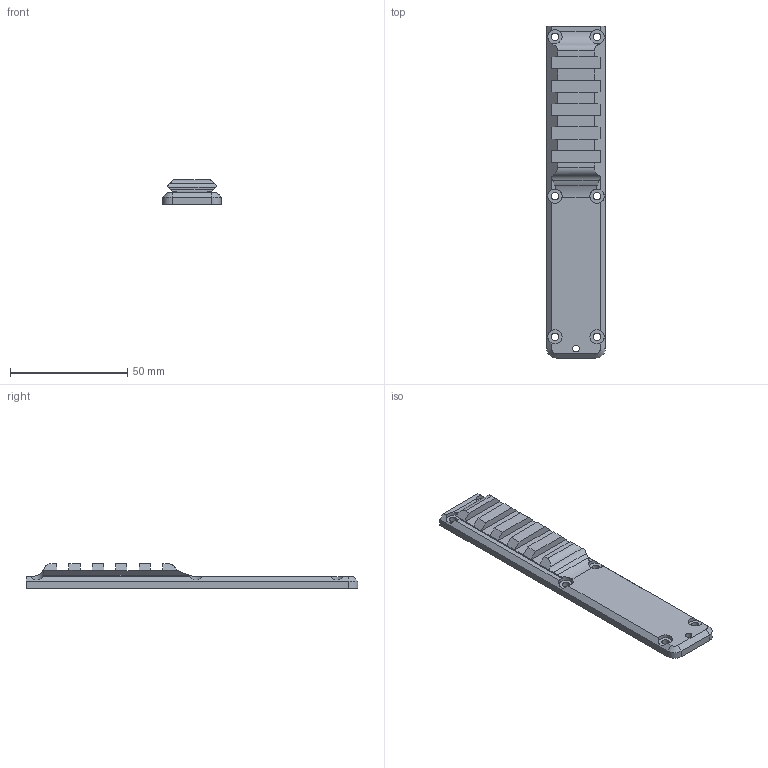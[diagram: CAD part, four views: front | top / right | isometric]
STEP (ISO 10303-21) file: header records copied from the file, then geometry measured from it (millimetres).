
FILE_DESCRIPTION(/* description */ (''),/* implementation_level */ '2;1');
FILE_NAME(/* name */ 'Receiver-Top-Cover_Picatinny.stp',/* time_stamp */ '2020-10-15T21:28:55-05:00',/* author */ (''),/* organization */ (''),/* preprocessor_version */ 'ST-DEVELOPER v15.2',/* originating_system */ 'Autodesk Translator Framework v2.0.0.5431',/* authorisation */ '');
FILE_SCHEMA (('AUTOMOTIVE_DESIGN { 1 0 10303 214 3 1 1 }'));
Length unit declared in the file: centimetre
Products named in the file (1): Receiver-Top-Cover_Picatinny
Bounding box: 25 x 141.66 x 10.47 mm (x, y, z)
Volume: 16500.9 mm3; surface area: 10986.9 mm2
Topology: 1 solids, 1 shells, 88 faces, 264 edges, 178 vertices
Faces by surface type: plane 61, cylinder 25, cone 2
Full cylindrical faces by diameter (mm): 2.8 x1, 3.2 x6
Entity records: 3066 total; most frequent: CARTESIAN_POINT 592, ORIENTED_EDGE 514, DIRECTION 509, EDGE_CURVE 257, VERTEX_POINT 178, LINE 175, VECTOR 175, AXIS2_PLACEMENT_3D 167
